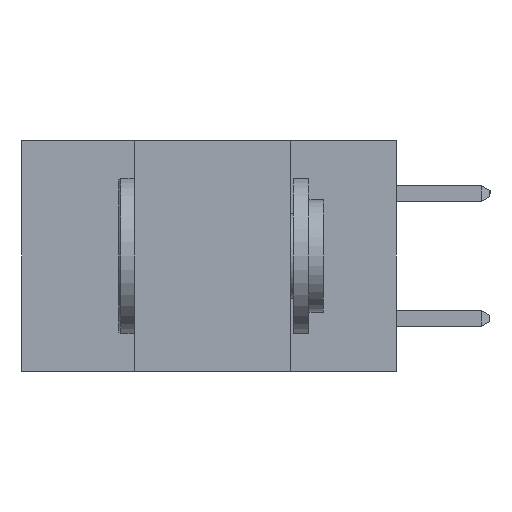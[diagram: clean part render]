
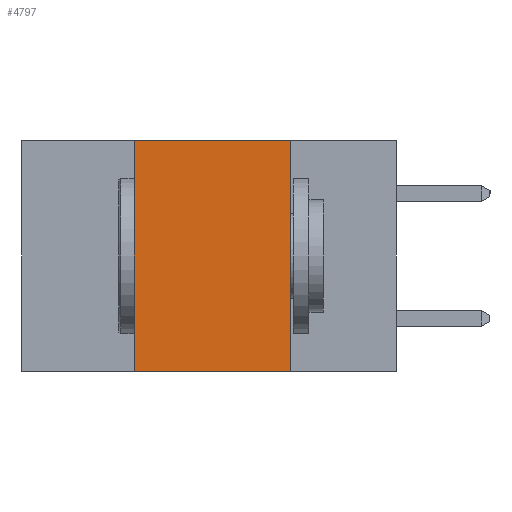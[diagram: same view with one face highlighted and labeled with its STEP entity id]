
A CAD part, left-side view. The second image highlights one B-rep face of the part: STEP entity #4797.
In plain terms, the highlighted planar face has unit normal (-1, 0, 0).
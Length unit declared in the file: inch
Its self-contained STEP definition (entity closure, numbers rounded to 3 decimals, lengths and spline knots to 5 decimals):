
#629 = CARTESIAN_POINT ( 'NONE',  ( 0., 0.42, 0. ) ) ;
#741 = DIRECTION ( 'NONE',  ( 0., -1., 0. ) ) ;
#1887 = ORIENTED_EDGE ( 'NONE', *, *, #9160, .F. ) ;
#2911 = VECTOR ( 'NONE', #8891, 39.37008 ) ;
#2929 = CARTESIAN_POINT ( 'NONE',  ( 0., 0.6, -0.37 ) ) ;
#3164 = EDGE_LOOP ( 'NONE', ( #6124, #1887, #6403, #8959 ) ) ;
#3657 = DIRECTION ( 'NONE',  ( 0., -1., 0. ) ) ;
#3996 = LINE ( 'NONE', #14043, #4157 ) ;
#4157 = VECTOR ( 'NONE', #11689, 39.37008 ) ;
#4797 = ADVANCED_FACE ( 'NONE', ( #6142 ), #7453, .F. ) ;
#5128 = DIRECTION ( 'NONE',  ( 1., 0., 0. ) ) ;
#5272 = VERTEX_POINT ( 'NONE', #10793 ) ;
#5505 = AXIS2_PLACEMENT_3D ( 'NONE', #7519, #5128, #11930 ) ;
#6001 = LINE ( 'NONE', #13702, #9243 ) ;
#6105 = VERTEX_POINT ( 'NONE', #9667 ) ;
#6124 = ORIENTED_EDGE ( 'NONE', *, *, #11515, .F. ) ;
#6142 = FACE_OUTER_BOUND ( 'NONE', #3164, .T. ) ;
#6403 = ORIENTED_EDGE ( 'NONE', *, *, #13943, .F. ) ;
#6891 = VECTOR ( 'NONE', #741, 39.37008 ) ;
#7453 = PLANE ( 'NONE',  #5505 ) ;
#7519 = CARTESIAN_POINT ( 'NONE',  ( 0., 0.6, 0. ) ) ;
#7587 = CARTESIAN_POINT ( 'NONE',  ( 0., 0.17, -0.37 ) ) ;
#7709 = CARTESIAN_POINT ( 'NONE',  ( 0., 0.42, -0.37 ) ) ;
#7867 = EDGE_CURVE ( 'NONE', #5272, #11894, #11500, .T. ) ;
#8891 = DIRECTION ( 'NONE',  ( 0., 0., 1. ) ) ;
#8959 = ORIENTED_EDGE ( 'NONE', *, *, #7867, .T. ) ;
#9160 = EDGE_CURVE ( 'NONE', #11512, #6105, #6001, .T. ) ;
#9243 = VECTOR ( 'NONE', #3657, 39.37008 ) ;
#9667 = CARTESIAN_POINT ( 'NONE',  ( 0., 0.17, 0. ) ) ;
#10793 = CARTESIAN_POINT ( 'NONE',  ( 0., 0.42, -0.37 ) ) ;
#11154 = LINE ( 'NONE', #7709, #2911 ) ;
#11500 = LINE ( 'NONE', #2929, #6891 ) ;
#11512 = VERTEX_POINT ( 'NONE', #629 ) ;
#11515 = EDGE_CURVE ( 'NONE', #6105, #11894, #3996, .T. ) ;
#11689 = DIRECTION ( 'NONE',  ( 0., 0., -1. ) ) ;
#11894 = VERTEX_POINT ( 'NONE', #7587 ) ;
#11930 = DIRECTION ( 'NONE',  ( 0., 0., -1. ) ) ;
#13702 = CARTESIAN_POINT ( 'NONE',  ( 0., 0.6, 0. ) ) ;
#13943 = EDGE_CURVE ( 'NONE', #5272, #11512, #11154, .T. ) ;
#14043 = CARTESIAN_POINT ( 'NONE',  ( 0., 0.17, -0.37 ) ) ;
